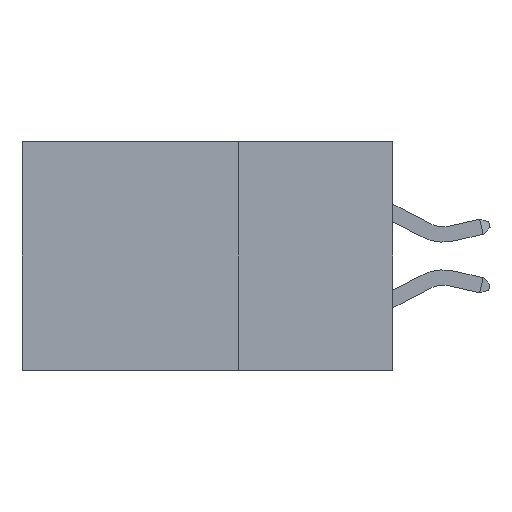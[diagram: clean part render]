
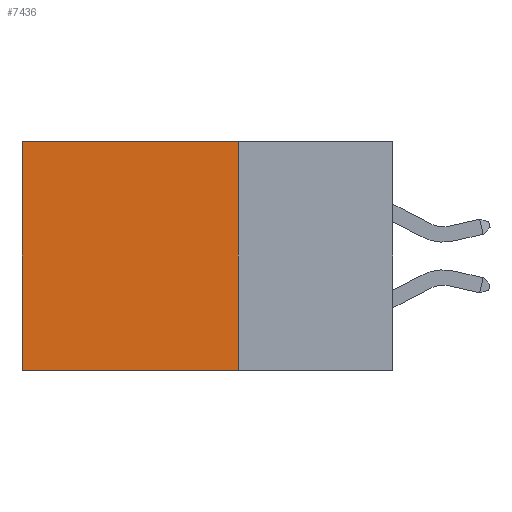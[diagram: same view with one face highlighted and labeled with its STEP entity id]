
A CAD part, left-side view. The second image highlights one B-rep face of the part: STEP entity #7436.
In plain terms, the highlighted planar face has unit normal (-1, 0, 0).
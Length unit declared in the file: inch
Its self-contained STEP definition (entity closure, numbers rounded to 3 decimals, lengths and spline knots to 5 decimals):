
#68 = VECTOR ( 'NONE', #4910, 39.37008 ) ;
#493 = DIRECTION ( 'NONE',  ( 0., 0., -1. ) ) ;
#632 = CARTESIAN_POINT ( 'NONE',  ( 0.2875, 0.6, 0. ) ) ;
#990 = EDGE_CURVE ( 'NONE', #9580, #13404, #2915, .T. ) ;
#995 = DIRECTION ( 'NONE',  ( 1., 0., 0. ) ) ;
#2143 = PLANE ( 'NONE',  #6903 ) ;
#2197 = VECTOR ( 'NONE', #10454, 39.37008 ) ;
#2915 = LINE ( 'NONE', #632, #10701 ) ;
#3547 = EDGE_CURVE ( 'NONE', #8052, #9580, #7486, .T. ) ;
#3928 = ORIENTED_EDGE ( 'NONE', *, *, #990, .T. ) ;
#4201 = CARTESIAN_POINT ( 'NONE',  ( 0.2875, 0.25, -0.37 ) ) ;
#4695 = ORIENTED_EDGE ( 'NONE', *, *, #3547, .T. ) ;
#4910 = DIRECTION ( 'NONE',  ( 0., 0., -1. ) ) ;
#5203 = CARTESIAN_POINT ( 'NONE',  ( 0.2875, 0.25, 0. ) ) ;
#6903 = AXIS2_PLACEMENT_3D ( 'NONE', #12653, #995, #8644 ) ;
#7246 = EDGE_CURVE ( 'NONE', #8052, #12310, #11499, .T. ) ;
#7266 = CARTESIAN_POINT ( 'NONE',  ( 0.2875, 0.6, 0. ) ) ;
#7288 = DIRECTION ( 'NONE',  ( 0., 1., 0. ) ) ;
#7436 = ADVANCED_FACE ( 'NONE', ( #13617 ), #2143, .F. ) ;
#7486 = LINE ( 'NONE', #5203, #12900 ) ;
#8052 = VERTEX_POINT ( 'NONE', #10885 ) ;
#8462 = EDGE_CURVE ( 'NONE', #12310, #13404, #12997, .T. ) ;
#8524 = ORIENTED_EDGE ( 'NONE', *, *, #8462, .F. ) ;
#8644 = DIRECTION ( 'NONE',  ( 0., 0., -1. ) ) ;
#9580 = VERTEX_POINT ( 'NONE', #7266 ) ;
#10454 = DIRECTION ( 'NONE',  ( 0., 1., 0. ) ) ;
#10701 = VECTOR ( 'NONE', #493, 39.37008 ) ;
#10885 = CARTESIAN_POINT ( 'NONE',  ( 0.2875, 0.25, 0. ) ) ;
#11051 = CARTESIAN_POINT ( 'NONE',  ( 0.2875, 0.25, -0.37 ) ) ;
#11499 = LINE ( 'NONE', #12113, #68 ) ;
#12113 = CARTESIAN_POINT ( 'NONE',  ( 0.2875, 0.25, 0. ) ) ;
#12310 = VERTEX_POINT ( 'NONE', #11051 ) ;
#12653 = CARTESIAN_POINT ( 'NONE',  ( 0.2875, 0.25, 0. ) ) ;
#12692 = ORIENTED_EDGE ( 'NONE', *, *, #7246, .F. ) ;
#12900 = VECTOR ( 'NONE', #7288, 39.37008 ) ;
#12963 = CARTESIAN_POINT ( 'NONE',  ( 0.2875, 0.6, -0.37 ) ) ;
#12997 = LINE ( 'NONE', #4201, #2197 ) ;
#13297 = EDGE_LOOP ( 'NONE', ( #3928, #8524, #12692, #4695 ) ) ;
#13404 = VERTEX_POINT ( 'NONE', #12963 ) ;
#13617 = FACE_OUTER_BOUND ( 'NONE', #13297, .T. ) ;
